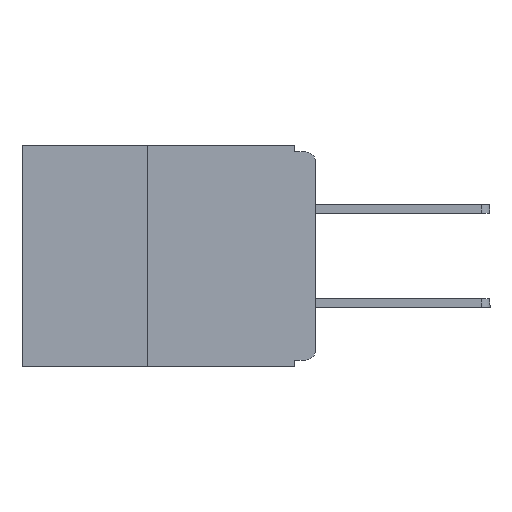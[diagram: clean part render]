
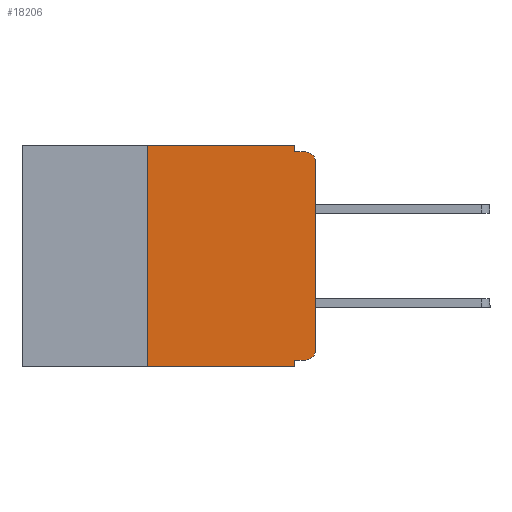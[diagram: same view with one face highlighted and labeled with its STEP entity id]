
A CAD part, left-side view. The second image highlights one B-rep face of the part: STEP entity #18206.
In plain terms, the highlighted planar face has unit normal (-1, 0, 0).
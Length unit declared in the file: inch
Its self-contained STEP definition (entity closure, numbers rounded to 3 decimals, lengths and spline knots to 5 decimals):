
#77 = LINE ( 'NONE', #8684, #3876 ) ;
#588 = VERTEX_POINT ( 'NONE', #17958 ) ;
#695 = CARTESIAN_POINT ( 'NONE',  ( 0., 0.015, -0.025 ) ) ;
#750 = CARTESIAN_POINT ( 'NONE',  ( 0., 0., 0. ) ) ;
#1220 = CARTESIAN_POINT ( 'NONE',  ( 0., 0., -0.32 ) ) ;
#1325 = EDGE_CURVE ( 'NONE', #588, #8035, #16174, .T. ) ;
#1342 = LINE ( 'NONE', #1220, #8601 ) ;
#1608 = LINE ( 'NONE', #6556, #5043 ) ;
#1972 = CARTESIAN_POINT ( 'NONE',  ( 0., 0., -0.305 ) ) ;
#2519 = CIRCLE ( 'NONE', #10732, 0.015 ) ;
#3358 = ORIENTED_EDGE ( 'NONE', *, *, #1325, .T. ) ;
#3363 = FACE_OUTER_BOUND ( 'NONE', #10737, .T. ) ;
#3814 = EDGE_CURVE ( 'NONE', #11930, #12888, #1608, .T. ) ;
#3876 = VECTOR ( 'NONE', #8267, 39.37008 ) ;
#3960 = DIRECTION ( 'NONE',  ( 0., -1., 0. ) ) ;
#3975 = CARTESIAN_POINT ( 'NONE',  ( 0., 0., -0.01 ) ) ;
#4276 = EDGE_CURVE ( 'NONE', #6283, #6768, #2519, .T. ) ;
#4533 = VERTEX_POINT ( 'NONE', #10604 ) ;
#4698 = ORIENTED_EDGE ( 'NONE', *, *, #8767, .F. ) ;
#4849 = ORIENTED_EDGE ( 'NONE', *, *, #9993, .F. ) ;
#4996 = EDGE_CURVE ( 'NONE', #4533, #13636, #10342, .T. ) ;
#5029 = VECTOR ( 'NONE', #10879, 39.37008 ) ;
#5036 = CARTESIAN_POINT ( 'NONE',  ( 0., 0.015, -0.01 ) ) ;
#5043 = VECTOR ( 'NONE', #12231, 39.37008 ) ;
#5590 = CARTESIAN_POINT ( 'NONE',  ( 0., 0.437, -0.33 ) ) ;
#5652 = AXIS2_PLACEMENT_3D ( 'NONE', #11372, #7058, #17038 ) ;
#6219 = CARTESIAN_POINT ( 'NONE',  ( 0., 0.015, -0.32 ) ) ;
#6283 = VERTEX_POINT ( 'NONE', #6219 ) ;
#6556 = CARTESIAN_POINT ( 'NONE',  ( 0., 0.25, -0.33 ) ) ;
#6768 = VERTEX_POINT ( 'NONE', #1972 ) ;
#6797 = LINE ( 'NONE', #6925, #7261 ) ;
#6925 = CARTESIAN_POINT ( 'NONE',  ( 0., 0.437, 0. ) ) ;
#7058 = DIRECTION ( 'NONE',  ( 1., 0., 0. ) ) ;
#7131 = VERTEX_POINT ( 'NONE', #11818 ) ;
#7261 = VECTOR ( 'NONE', #15564, 39.37008 ) ;
#8035 = VERTEX_POINT ( 'NONE', #5036 ) ;
#8267 = DIRECTION ( 'NONE',  ( 0., 0., -1. ) ) ;
#8554 = DIRECTION ( 'NONE',  ( 0., -1., 0. ) ) ;
#8579 = EDGE_CURVE ( 'NONE', #6768, #588, #8855, .T. ) ;
#8601 = VECTOR ( 'NONE', #11398, 39.37008 ) ;
#8684 = CARTESIAN_POINT ( 'NONE',  ( 0., 0.031, 0. ) ) ;
#8767 = EDGE_CURVE ( 'NONE', #9421, #8035, #17531, .T. ) ;
#8812 = VECTOR ( 'NONE', #8554, 39.37008 ) ;
#8855 = LINE ( 'NONE', #750, #5029 ) ;
#8883 = EDGE_CURVE ( 'NONE', #7131, #9421, #77, .T. ) ;
#9421 = VERTEX_POINT ( 'NONE', #13109 ) ;
#9547 = VECTOR ( 'NONE', #3960, 39.37008 ) ;
#9651 = CARTESIAN_POINT ( 'NONE',  ( 0., 0.031, -0.33 ) ) ;
#9993 = EDGE_CURVE ( 'NONE', #6283, #4533, #1342, .T. ) ;
#10290 = ORIENTED_EDGE ( 'NONE', *, *, #13805, .T. ) ;
#10342 = LINE ( 'NONE', #18347, #17019 ) ;
#10604 = CARTESIAN_POINT ( 'NONE',  ( 0., 0.031, -0.32 ) ) ;
#10732 = AXIS2_PLACEMENT_3D ( 'NONE', #16648, #16565, #16587 ) ;
#10737 = EDGE_LOOP ( 'NONE', ( #13361, #3358, #4698, #17866, #11027, #15593, #10290, #13987, #4849, #14351 ) ) ;
#10879 = DIRECTION ( 'NONE',  ( 0., 0., 1. ) ) ;
#11027 = ORIENTED_EDGE ( 'NONE', *, *, #13713, .F. ) ;
#11310 = DIRECTION ( 'NONE',  ( 0., 0., -1. ) ) ;
#11372 = CARTESIAN_POINT ( 'NONE',  ( 0., 0.437, 0. ) ) ;
#11398 = DIRECTION ( 'NONE',  ( 0., 1., 0. ) ) ;
#11818 = CARTESIAN_POINT ( 'NONE',  ( 0., 0.031, 0. ) ) ;
#11930 = VERTEX_POINT ( 'NONE', #15963 ) ;
#12231 = DIRECTION ( 'NONE',  ( 0., 0., 1. ) ) ;
#12682 = LINE ( 'NONE', #5590, #8812 ) ;
#12888 = VERTEX_POINT ( 'NONE', #15123 ) ;
#13109 = CARTESIAN_POINT ( 'NONE',  ( 0., 0.031, -0.01 ) ) ;
#13361 = ORIENTED_EDGE ( 'NONE', *, *, #8579, .T. ) ;
#13636 = VERTEX_POINT ( 'NONE', #9651 ) ;
#13713 = EDGE_CURVE ( 'NONE', #12888, #7131, #6797, .T. ) ;
#13759 = DIRECTION ( 'NONE',  ( -1., 0., 0. ) ) ;
#13805 = EDGE_CURVE ( 'NONE', #11930, #13636, #12682, .T. ) ;
#13987 = ORIENTED_EDGE ( 'NONE', *, *, #4996, .F. ) ;
#14351 = ORIENTED_EDGE ( 'NONE', *, *, #4276, .T. ) ;
#15123 = CARTESIAN_POINT ( 'NONE',  ( 0., 0.25, 0. ) ) ;
#15304 = AXIS2_PLACEMENT_3D ( 'NONE', #695, #13759, #11310 ) ;
#15564 = DIRECTION ( 'NONE',  ( 0., -1., 0. ) ) ;
#15593 = ORIENTED_EDGE ( 'NONE', *, *, #3814, .F. ) ;
#15700 = PLANE ( 'NONE',  #5652 ) ;
#15963 = CARTESIAN_POINT ( 'NONE',  ( 0., 0.25, -0.33 ) ) ;
#16174 = CIRCLE ( 'NONE', #15304, 0.015 ) ;
#16565 = DIRECTION ( 'NONE',  ( -1., 0., 0. ) ) ;
#16587 = DIRECTION ( 'NONE',  ( 0., 0., -1. ) ) ;
#16648 = CARTESIAN_POINT ( 'NONE',  ( 0., 0.015, -0.305 ) ) ;
#17019 = VECTOR ( 'NONE', #18383, 39.37008 ) ;
#17038 = DIRECTION ( 'NONE',  ( 0., 0., -1. ) ) ;
#17531 = LINE ( 'NONE', #3975, #9547 ) ;
#17866 = ORIENTED_EDGE ( 'NONE', *, *, #8883, .F. ) ;
#17958 = CARTESIAN_POINT ( 'NONE',  ( 0., 0., -0.025 ) ) ;
#18206 = ADVANCED_FACE ( 'NONE', ( #3363 ), #15700, .F. ) ;
#18347 = CARTESIAN_POINT ( 'NONE',  ( 0., 0.031, -0.33 ) ) ;
#18383 = DIRECTION ( 'NONE',  ( 0., 0., -1. ) ) ;
